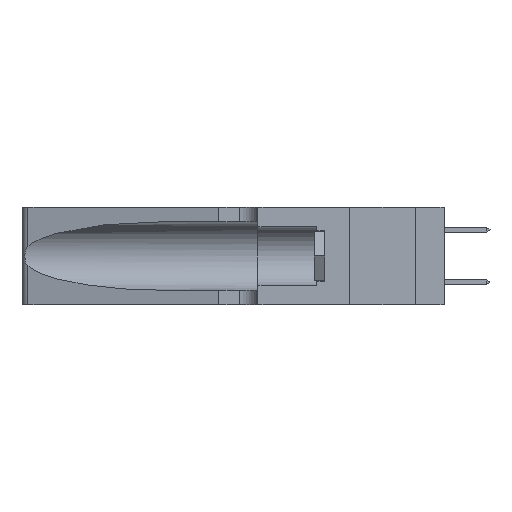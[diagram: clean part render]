
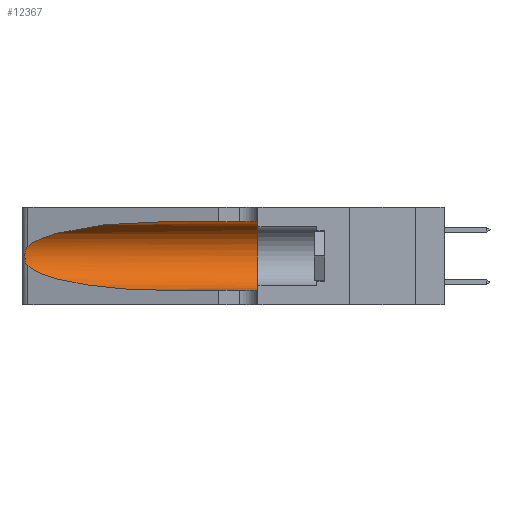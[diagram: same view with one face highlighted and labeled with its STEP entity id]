
A CAD part, left-side view. The second image highlights one B-rep face of the part: STEP entity #12367.
In plain terms, the highlighted cylindrical face has radius 3.308 mm (diameter 6.617 mm), a partial arc.
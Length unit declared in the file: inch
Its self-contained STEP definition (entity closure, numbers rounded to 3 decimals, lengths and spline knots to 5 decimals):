
#228 = FACE_OUTER_BOUND ( 'NONE', #19001, .T. ) ;
#380 = CARTESIAN_POINT ( 'NONE',  ( 0.1305, 0.72297, 0.05475 ) ) ;
#516 = ORIENTED_EDGE ( 'NONE', *, *, #13768, .T. ) ;
#871 = CARTESIAN_POINT ( 'NONE',  ( 0.1305, 1.61858, 0.185 ) ) ;
#1123 = CARTESIAN_POINT ( 'NONE',  ( 0.1305, 0.35, 0.185 ) ) ;
#1201 = CARTESIAN_POINT ( 'NONE',  ( 0.25789, 1.23486, 0.15765 ) ) ;
#1258 = CARTESIAN_POINT ( 'NONE',  ( 0.25555, 1.22993, 0.14849 ) ) ;
#1989 = LINE ( 'NONE', #3608, #13814 ) ;
#2241 = VERTEX_POINT ( 'NONE', #9832 ) ;
#2461 = DIRECTION ( 'NONE',  ( 0., 0., 1. ) ) ;
#2608 = CARTESIAN_POINT ( 'NONE',  ( 0.25555, 1.22994, 0.2215 ) ) ;
#3102 = CARTESIAN_POINT ( 'NONE',  ( 0.25487, 1.22718, 0.14631 ) ) ;
#3395 = CARTESIAN_POINT ( 'NONE',  ( 0.1305, 0.72297, 0.05475 ) ) ;
#3582 = DIRECTION ( 'NONE',  ( 0., -1., 0. ) ) ;
#3608 = CARTESIAN_POINT ( 'NONE',  ( 0.1305, 1.61858, 0.31525 ) ) ;
#3648 = B_SPLINE_CURVE_WITH_KNOTS ( 'NONE', 3,
 ( #5726, #2608, #18833, #13177, #7185, #18904, #10280, #8810, #13240, #10069, #1201, #10146, #1258, #10410 ),
 .UNSPECIFIED., .F., .F.,
 ( 4, 2, 2, 2, 2, 2, 4 ),
 ( 0., 0.00027, 0.00053, 0.00107, 0.0016, 0.00187, 0.00214 ),
 .UNSPECIFIED. ) ;
#4311 = CARTESIAN_POINT ( 'NONE',  ( 0.25487, 1.22718, 0.22369 ) ) ;
#4944 = VERTEX_POINT ( 'NONE', #6935 ) ;
#5125 = CARTESIAN_POINT ( 'NONE',  ( 0.1305, 1.61858, 0.05475 ) ) ;
#5550 = EDGE_CURVE ( 'NONE', #4944, #12976, #6514, .T. ) ;
#5726 = CARTESIAN_POINT ( 'NONE',  ( 0.25487, 1.22718, 0.22369 ) ) ;
#6514 =( BOUNDED_CURVE ( )  B_SPLINE_CURVE ( 3, ( #13890, #14011, #10475, #4311 ),
 .UNSPECIFIED., .F., .T. ) 
 B_SPLINE_CURVE_WITH_KNOTS ( ( 4, 4 ),
 ( 1.5708, 2.84003 ),
 .UNSPECIFIED. ) 
 CURVE ( )  GEOMETRIC_REPRESENTATION_ITEM ( )  RATIONAL_B_SPLINE_CURVE ( ( 1., 0.87, 0.87, 1. ) ) 
 REPRESENTATION_ITEM ( '' )  );
#6935 = CARTESIAN_POINT ( 'NONE',  ( 0.1305, 0.72297, 0.31525 ) ) ;
#7185 = CARTESIAN_POINT ( 'NONE',  ( 0.25854, 1.2359, 0.20912 ) ) ;
#7713 = CARTESIAN_POINT ( 'NONE',  ( 0.2373, 1.15595, 0.08982 ) ) ;
#7820 = ORIENTED_EDGE ( 'NONE', *, *, #5550, .T. ) ;
#7871 = VERTEX_POINT ( 'NONE', #17467 ) ;
#8459 = VERTEX_POINT ( 'NONE', #17045 ) ;
#8810 = CARTESIAN_POINT ( 'NONE',  ( 0.26075, 1.23896, 0.178 ) ) ;
#9517 = ORIENTED_EDGE ( 'NONE', *, *, #10576, .T. ) ;
#9803 = LINE ( 'NONE', #5125, #11196 ) ;
#9832 = CARTESIAN_POINT ( 'NONE',  ( 0.1305, 0.35, 0.31525 ) ) ;
#10069 = CARTESIAN_POINT ( 'NONE',  ( 0.25856, 1.23593, 0.16098 ) ) ;
#10146 = CARTESIAN_POINT ( 'NONE',  ( 0.25639, 1.23186, 0.15144 ) ) ;
#10280 = CARTESIAN_POINT ( 'NONE',  ( 0.26075, 1.23896, 0.19203 ) ) ;
#10338 = ORIENTED_EDGE ( 'NONE', *, *, #11125, .T. ) ;
#10410 = CARTESIAN_POINT ( 'NONE',  ( 0.25487, 1.22718, 0.14631 ) ) ;
#10475 = CARTESIAN_POINT ( 'NONE',  ( 0.2373, 1.15595, 0.28018 ) ) ;
#10576 = EDGE_CURVE ( 'NONE', #13903, #8459, #9803, .T. ) ;
#11060 = DIRECTION ( 'NONE',  ( 0., -1., 0. ) ) ;
#11125 = EDGE_CURVE ( 'NONE', #12976, #7871, #3648, .T. ) ;
#11196 = VECTOR ( 'NONE', #15474, 39.37008 ) ;
#12252 = CYLINDRICAL_SURFACE ( 'NONE', #14804, 0.13025 ) ;
#12367 = ADVANCED_FACE ( 'NONE', ( #228 ), #12252, .F. ) ;
#12526 = CARTESIAN_POINT ( 'NONE',  ( 0.25487, 1.22718, 0.22369 ) ) ;
#12545 =( BOUNDED_CURVE ( )  B_SPLINE_CURVE ( 3, ( #3102, #7713, #13764, #380 ),
 .UNSPECIFIED., .F., .T. ) 
 B_SPLINE_CURVE_WITH_KNOTS ( ( 4, 4 ),
 ( 3.44316, 4.71239 ),
 .UNSPECIFIED. ) 
 CURVE ( )  GEOMETRIC_REPRESENTATION_ITEM ( )  RATIONAL_B_SPLINE_CURVE ( ( 1., 0.87, 0.87, 1. ) ) 
 REPRESENTATION_ITEM ( '' )  );
#12664 = CIRCLE ( 'NONE', #18042, 0.13025 ) ;
#12976 = VERTEX_POINT ( 'NONE', #12526 ) ;
#13177 = CARTESIAN_POINT ( 'NONE',  ( 0.25787, 1.23484, 0.2124 ) ) ;
#13240 = CARTESIAN_POINT ( 'NONE',  ( 0.26017, 1.23833, 0.17102 ) ) ;
#13252 = ORIENTED_EDGE ( 'NONE', *, *, #15007, .F. ) ;
#13764 = CARTESIAN_POINT ( 'NONE',  ( 0.18966, 0.96281, 0.05475 ) ) ;
#13768 = EDGE_CURVE ( 'NONE', #7871, #13903, #12545, .T. ) ;
#13814 = VECTOR ( 'NONE', #11060, 39.37008 ) ;
#13890 = CARTESIAN_POINT ( 'NONE',  ( 0.1305, 0.72297, 0.31525 ) ) ;
#13903 = VERTEX_POINT ( 'NONE', #3395 ) ;
#14011 = CARTESIAN_POINT ( 'NONE',  ( 0.18966, 0.96281, 0.31525 ) ) ;
#14703 = EDGE_CURVE ( 'NONE', #2241, #8459, #12664, .T. ) ;
#14804 = AXIS2_PLACEMENT_3D ( 'NONE', #871, #3582, #15413 ) ;
#15007 = EDGE_CURVE ( 'NONE', #4944, #2241, #1989, .T. ) ;
#15413 = DIRECTION ( 'NONE',  ( 0., 0., -1. ) ) ;
#15474 = DIRECTION ( 'NONE',  ( 0., -1., 0. ) ) ;
#15844 = ORIENTED_EDGE ( 'NONE', *, *, #14703, .F. ) ;
#17045 = CARTESIAN_POINT ( 'NONE',  ( 0.1305, 0.35, 0.05475 ) ) ;
#17467 = CARTESIAN_POINT ( 'NONE',  ( 0.25487, 1.22718, 0.14631 ) ) ;
#18042 = AXIS2_PLACEMENT_3D ( 'NONE', #1123, #18820, #2461 ) ;
#18820 = DIRECTION ( 'NONE',  ( 0., 1., 0. ) ) ;
#18833 = CARTESIAN_POINT ( 'NONE',  ( 0.25639, 1.23184, 0.21858 ) ) ;
#18904 = CARTESIAN_POINT ( 'NONE',  ( 0.26018, 1.23835, 0.19895 ) ) ;
#19001 = EDGE_LOOP ( 'NONE', ( #7820, #10338, #516, #9517, #15844, #13252 ) ) ;
